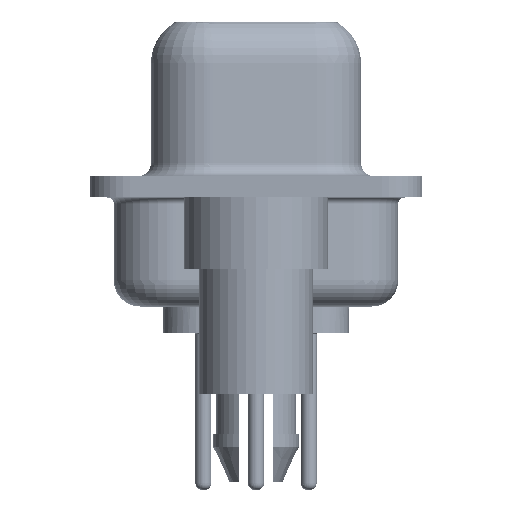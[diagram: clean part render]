
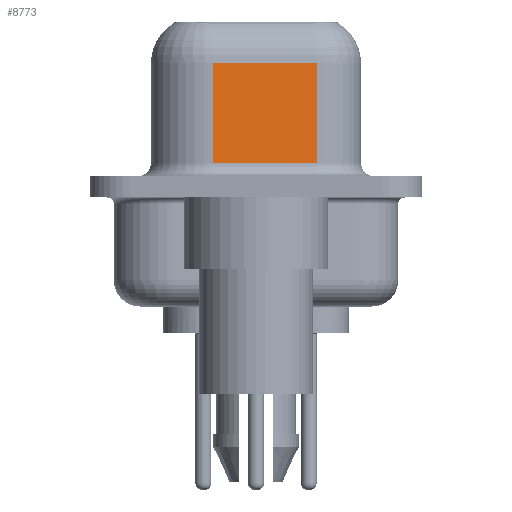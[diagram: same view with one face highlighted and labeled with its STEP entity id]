
A CAD part, left-side view. The second image highlights one B-rep face of the part: STEP entity #8773.
In plain terms, the highlighted planar face has unit normal (-0.985, -0.174, 0).
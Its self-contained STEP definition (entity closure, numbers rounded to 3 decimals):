
#554 = EDGE_CURVE ( 'NONE', #9674, #30265, #27966, .T. ) ;
#1352 = CARTESIAN_POINT ( 'NONE',  ( 5.068, -2.297, 4.65 ) ) ;
#2466 = AXIS2_PLACEMENT_3D ( 'NONE', #35007, #20901, #23653 ) ;
#2986 = DIRECTION ( 'NONE',  ( 0.174, -0.985, 0. ) ) ;
#3217 = CARTESIAN_POINT ( 'NONE',  ( 4.38, 1.603, 0.9 ) ) ;
#4340 = LINE ( 'NONE', #25279, #21830 ) ;
#4766 = VECTOR ( 'NONE', #35745, 1000. ) ;
#8067 = ORIENTED_EDGE ( 'NONE', *, *, #23387, .T. ) ;
#8773 = ADVANCED_FACE ( 'NONE', ( #38135 ), #26209, .F. ) ;
#9674 = VERTEX_POINT ( 'NONE', #24973 ) ;
#11068 = CARTESIAN_POINT ( 'NONE',  ( 4.38, 1.603, 6.4 ) ) ;
#11136 = DIRECTION ( 'NONE',  ( 0., 0., -1. ) ) ;
#12629 = VECTOR ( 'NONE', #25633, 1000. ) ;
#12857 = VERTEX_POINT ( 'NONE', #32739 ) ;
#13481 = VERTEX_POINT ( 'NONE', #3217 ) ;
#14277 = ORIENTED_EDGE ( 'NONE', *, *, #554, .T. ) ;
#17197 = EDGE_CURVE ( 'NONE', #9674, #12857, #4340, .T. ) ;
#17722 = LINE ( 'NONE', #11068, #4766 ) ;
#18908 = EDGE_LOOP ( 'NONE', ( #32703, #14277, #8067, #34244 ) ) ;
#20901 = DIRECTION ( 'NONE',  ( 0.985, 0.174, 0. ) ) ;
#21830 = VECTOR ( 'NONE', #11136, 1000. ) ;
#23387 = EDGE_CURVE ( 'NONE', #30265, #13481, #17722, .T. ) ;
#23653 = DIRECTION ( 'NONE',  ( -0.174, 0.985, 0. ) ) ;
#24120 = LINE ( 'NONE', #36449, #29207 ) ;
#24973 = CARTESIAN_POINT ( 'NONE',  ( 5.068, -2.297, 4.65 ) ) ;
#25279 = CARTESIAN_POINT ( 'NONE',  ( 5.068, -2.297, 6.4 ) ) ;
#25633 = DIRECTION ( 'NONE',  ( -0.174, 0.985, 0. ) ) ;
#26209 = PLANE ( 'NONE',  #2466 ) ;
#27966 = LINE ( 'NONE', #1352, #12629 ) ;
#29207 = VECTOR ( 'NONE', #2986, 1000. ) ;
#30265 = VERTEX_POINT ( 'NONE', #33793 ) ;
#32703 = ORIENTED_EDGE ( 'NONE', *, *, #17197, .F. ) ;
#32739 = CARTESIAN_POINT ( 'NONE',  ( 5.068, -2.297, 0.9 ) ) ;
#33793 = CARTESIAN_POINT ( 'NONE',  ( 4.38, 1.603, 4.65 ) ) ;
#34244 = ORIENTED_EDGE ( 'NONE', *, *, #37884, .T. ) ;
#35007 = CARTESIAN_POINT ( 'NONE',  ( 5.068, -2.297, 6.4 ) ) ;
#35745 = DIRECTION ( 'NONE',  ( 0., 0., -1. ) ) ;
#36449 = CARTESIAN_POINT ( 'NONE',  ( 5.068, -2.297, 0.9 ) ) ;
#37884 = EDGE_CURVE ( 'NONE', #13481, #12857, #24120, .T. ) ;
#38135 = FACE_OUTER_BOUND ( 'NONE', #18908, .T. ) ;
